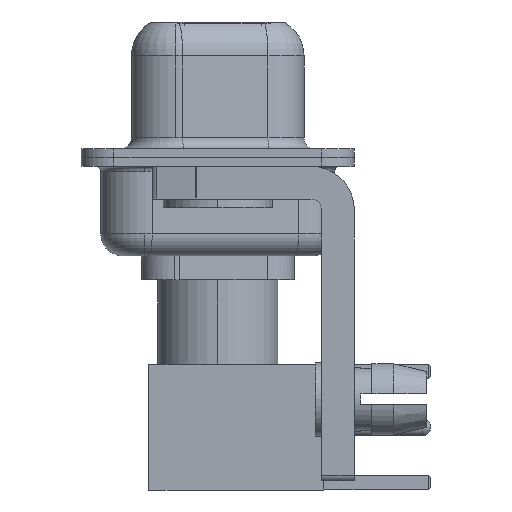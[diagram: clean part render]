
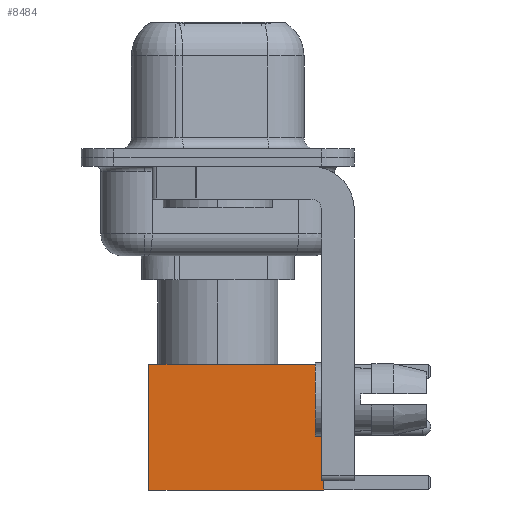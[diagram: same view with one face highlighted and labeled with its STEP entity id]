
A CAD part, left-side view. The second image highlights one B-rep face of the part: STEP entity #8484.
In plain terms, the highlighted face is planar.
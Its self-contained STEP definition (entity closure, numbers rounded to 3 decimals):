
#66 = ORIENTED_EDGE ( 'NONE', *, *, #10566, .F. ) ;
#519 = LINE ( 'NONE', #1745, #14425 ) ;
#838 = CARTESIAN_POINT ( 'NONE',  ( 2.875, 2.875, 8. ) ) ;
#1606 = ORIENTED_EDGE ( 'NONE', *, *, #15891, .T. ) ;
#1745 = CARTESIAN_POINT ( 'NONE',  ( 2.875, 2.875, 0. ) ) ;
#1867 = CARTESIAN_POINT ( 'NONE',  ( 2.875, 2.875, 0. ) ) ;
#1960 = PLANE ( 'NONE',  #15000 ) ;
#3222 = EDGE_CURVE ( 'NONE', #7917, #16221, #519, .T. ) ;
#3454 = DIRECTION ( 'NONE',  ( 0., 0., 1. ) ) ;
#4436 = ORIENTED_EDGE ( 'NONE', *, *, #3222, .T. ) ;
#5280 = LINE ( 'NONE', #10447, #7499 ) ;
#5695 = CARTESIAN_POINT ( 'NONE',  ( 0., 2.875, 8. ) ) ;
#6741 = ORIENTED_EDGE ( 'NONE', *, *, #13727, .F. ) ;
#7499 = VECTOR ( 'NONE', #17446, 1000. ) ;
#7554 = DIRECTION ( 'NONE',  ( 0., 1., 0. ) ) ;
#7789 = VECTOR ( 'NONE', #14786, 1000. ) ;
#7917 = VERTEX_POINT ( 'NONE', #838 ) ;
#8484 = ADVANCED_FACE ( 'NONE', ( #16389 ), #1960, .T. ) ;
#9121 = LINE ( 'NONE', #13226, #7789 ) ;
#10447 = CARTESIAN_POINT ( 'NONE',  ( 0., 2.875, 0. ) ) ;
#10566 = EDGE_CURVE ( 'NONE', #7917, #10585, #11271, .T. ) ;
#10585 = VERTEX_POINT ( 'NONE', #12855 ) ;
#11261 = DIRECTION ( 'NONE',  ( -1., 0., 0. ) ) ;
#11271 = LINE ( 'NONE', #5695, #16921 ) ;
#12590 = CARTESIAN_POINT ( 'NONE',  ( 2.875, 2.875, 0. ) ) ;
#12855 = CARTESIAN_POINT ( 'NONE',  ( -2.875, 2.875, 8. ) ) ;
#13106 = DIRECTION ( 'NONE',  ( 0., 0., -1. ) ) ;
#13226 = CARTESIAN_POINT ( 'NONE',  ( -2.875, 2.875, 0. ) ) ;
#13578 = VERTEX_POINT ( 'NONE', #17422 ) ;
#13727 = EDGE_CURVE ( 'NONE', #10585, #13578, #9121, .T. ) ;
#14268 = EDGE_LOOP ( 'NONE', ( #4436, #1606, #6741, #66 ) ) ;
#14425 = VECTOR ( 'NONE', #13106, 1000. ) ;
#14786 = DIRECTION ( 'NONE',  ( 0., 0., -1. ) ) ;
#15000 = AXIS2_PLACEMENT_3D ( 'NONE', #1867, #7554, #3454 ) ;
#15891 = EDGE_CURVE ( 'NONE', #16221, #13578, #5280, .T. ) ;
#16221 = VERTEX_POINT ( 'NONE', #12590 ) ;
#16389 = FACE_OUTER_BOUND ( 'NONE', #14268, .T. ) ;
#16921 = VECTOR ( 'NONE', #11261, 1000. ) ;
#17422 = CARTESIAN_POINT ( 'NONE',  ( -2.875, 2.875, 0. ) ) ;
#17446 = DIRECTION ( 'NONE',  ( -1., 0., 0. ) ) ;
